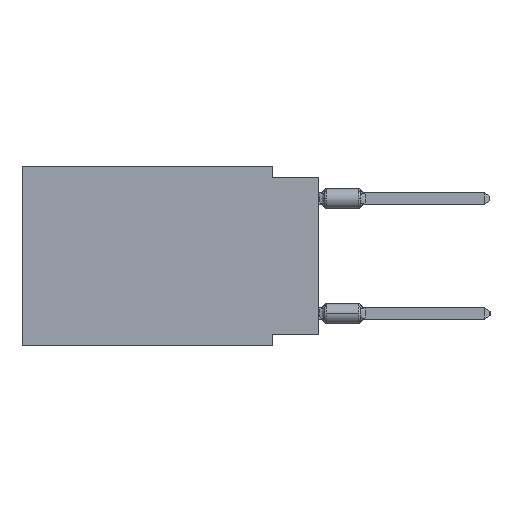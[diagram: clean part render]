
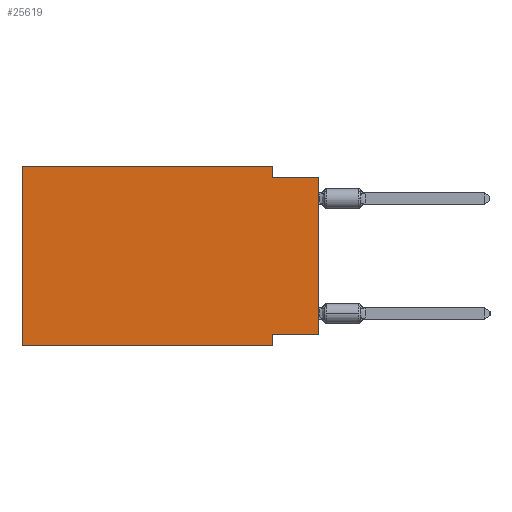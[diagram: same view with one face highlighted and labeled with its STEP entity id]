
A CAD part, left-side view. The second image highlights one B-rep face of the part: STEP entity #25619.
In plain terms, the highlighted planar face has unit normal (-1, 0, 0).
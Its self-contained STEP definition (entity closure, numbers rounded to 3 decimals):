
#322 = EDGE_CURVE ( 'NONE', #12493, #25074, #13907, .T. ) ;
#1152 = DIRECTION ( 'NONE',  ( 0., 0., -1. ) ) ;
#1393 = VERTEX_POINT ( 'NONE', #23640 ) ;
#1675 = FACE_OUTER_BOUND ( 'NONE', #18722, .T. ) ;
#1892 = VECTOR ( 'NONE', #5062, 1000. ) ;
#1893 = CARTESIAN_POINT ( 'NONE',  ( 0., 16.383, 0. ) ) ;
#3787 = ORIENTED_EDGE ( 'NONE', *, *, #20475, .F. ) ;
#3930 = DIRECTION ( 'NONE',  ( 0., 0., -1. ) ) ;
#5062 = DIRECTION ( 'NONE',  ( 0., -1., 0. ) ) ;
#5114 = CARTESIAN_POINT ( 'NONE',  ( 0., 16.383, 0. ) ) ;
#5476 = CARTESIAN_POINT ( 'NONE',  ( 0., 0., -0.635 ) ) ;
#6713 = CARTESIAN_POINT ( 'NONE',  ( 0., 16.383, 0. ) ) ;
#7251 = DIRECTION ( 'NONE',  ( 1., 0., 0. ) ) ;
#8160 = DIRECTION ( 'NONE',  ( 0., 0., 1. ) ) ;
#8403 = LINE ( 'NONE', #19570, #1892 ) ;
#8566 = ORIENTED_EDGE ( 'NONE', *, *, #22904, .T. ) ;
#9711 = VERTEX_POINT ( 'NONE', #21639 ) ;
#10692 = DIRECTION ( 'NONE',  ( 0., -1., 0. ) ) ;
#11063 = LINE ( 'NONE', #5476, #20800 ) ;
#12299 = DIRECTION ( 'NONE',  ( 0., 0., -1. ) ) ;
#12493 = VERTEX_POINT ( 'NONE', #20163 ) ;
#13014 = PLANE ( 'NONE',  #23446 ) ;
#13907 = LINE ( 'NONE', #18943, #24154 ) ;
#14852 = ORIENTED_EDGE ( 'NONE', *, *, #29833, .F. ) ;
#16985 = ORIENTED_EDGE ( 'NONE', *, *, #30568, .F. ) ;
#17762 = VERTEX_POINT ( 'NONE', #30278 ) ;
#18657 = ORIENTED_EDGE ( 'NONE', *, *, #322, .T. ) ;
#18722 = EDGE_LOOP ( 'NONE', ( #18657, #3787, #22400, #29832, #29362, #8566, #16985, #14852 ) ) ;
#18943 = CARTESIAN_POINT ( 'NONE',  ( 0., 0., 0. ) ) ;
#19227 = EDGE_CURVE ( 'NONE', #20516, #9711, #27394, .T. ) ;
#19246 = CARTESIAN_POINT ( 'NONE',  ( 0., 16.383, -9.906 ) ) ;
#19410 = EDGE_CURVE ( 'NONE', #9711, #1393, #29415, .T. ) ;
#19570 = CARTESIAN_POINT ( 'NONE',  ( 0., 16.383, -9.906 ) ) ;
#19818 = CARTESIAN_POINT ( 'NONE',  ( 0., 0., -0.635 ) ) ;
#20163 = CARTESIAN_POINT ( 'NONE',  ( 0., 0., -9.271 ) ) ;
#20475 = EDGE_CURVE ( 'NONE', #1393, #25074, #11063, .T. ) ;
#20516 = VERTEX_POINT ( 'NONE', #5114 ) ;
#20682 = LINE ( 'NONE', #6713, #29163 ) ;
#20800 = VECTOR ( 'NONE', #10692, 1000. ) ;
#21222 = EDGE_CURVE ( 'NONE', #36142, #20516, #20682, .T. ) ;
#21603 = LINE ( 'NONE', #27206, #27046 ) ;
#21639 = CARTESIAN_POINT ( 'NONE',  ( 0., 2.54, 0. ) ) ;
#22400 = ORIENTED_EDGE ( 'NONE', *, *, #19410, .F. ) ;
#22902 = VECTOR ( 'NONE', #33163, 1000. ) ;
#22904 = EDGE_CURVE ( 'NONE', #36142, #23459, #8403, .T. ) ;
#23446 = AXIS2_PLACEMENT_3D ( 'NONE', #32575, #7251, #3930 ) ;
#23459 = VERTEX_POINT ( 'NONE', #34356 ) ;
#23471 = CARTESIAN_POINT ( 'NONE',  ( 0., 2.54, 0. ) ) ;
#23640 = CARTESIAN_POINT ( 'NONE',  ( 0., 2.54, -0.635 ) ) ;
#24154 = VECTOR ( 'NONE', #8160, 1000. ) ;
#25074 = VERTEX_POINT ( 'NONE', #19818 ) ;
#25619 = ADVANCED_FACE ( 'NONE', ( #1675 ), #13014, .F. ) ;
#26801 = DIRECTION ( 'NONE',  ( 0., 0., 1. ) ) ;
#27005 = CARTESIAN_POINT ( 'NONE',  ( 0., 2.54, -9.906 ) ) ;
#27046 = VECTOR ( 'NONE', #29972, 1000. ) ;
#27206 = CARTESIAN_POINT ( 'NONE',  ( 0., 0., -9.271 ) ) ;
#27394 = LINE ( 'NONE', #1893, #22902 ) ;
#27591 = VECTOR ( 'NONE', #1152, 1000. ) ;
#29163 = VECTOR ( 'NONE', #26801, 1000. ) ;
#29362 = ORIENTED_EDGE ( 'NONE', *, *, #21222, .F. ) ;
#29415 = LINE ( 'NONE', #23471, #36599 ) ;
#29832 = ORIENTED_EDGE ( 'NONE', *, *, #19227, .F. ) ;
#29833 = EDGE_CURVE ( 'NONE', #12493, #17762, #21603, .T. ) ;
#29972 = DIRECTION ( 'NONE',  ( 0., 1., 0. ) ) ;
#30278 = CARTESIAN_POINT ( 'NONE',  ( 0., 2.54, -9.271 ) ) ;
#30568 = EDGE_CURVE ( 'NONE', #17762, #23459, #32767, .T. ) ;
#32575 = CARTESIAN_POINT ( 'NONE',  ( 0., 16.383, 0. ) ) ;
#32767 = LINE ( 'NONE', #27005, #27591 ) ;
#33163 = DIRECTION ( 'NONE',  ( 0., -1., 0. ) ) ;
#34356 = CARTESIAN_POINT ( 'NONE',  ( 0., 2.54, -9.906 ) ) ;
#36142 = VERTEX_POINT ( 'NONE', #19246 ) ;
#36599 = VECTOR ( 'NONE', #12299, 1000. ) ;
